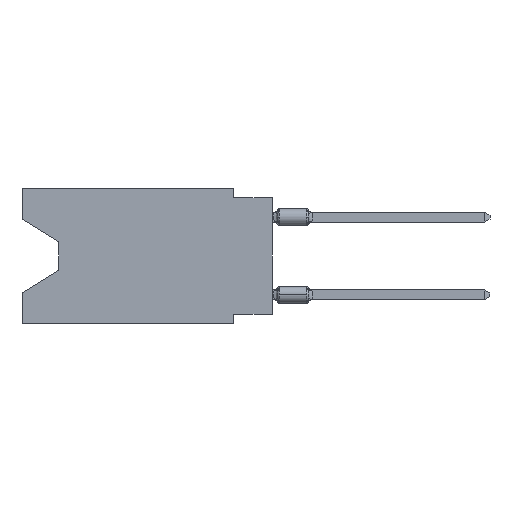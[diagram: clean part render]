
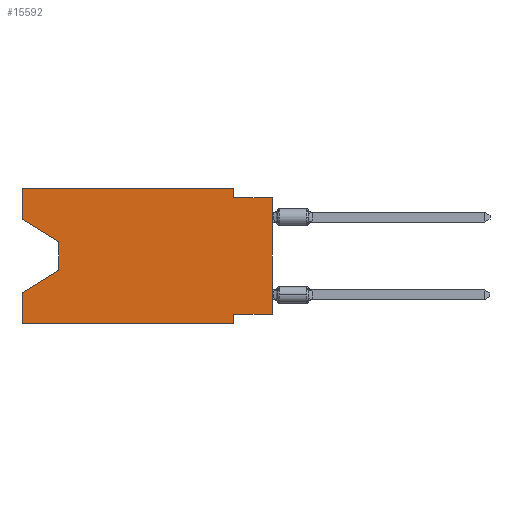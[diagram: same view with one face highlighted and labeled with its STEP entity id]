
A CAD part, left-side view. The second image highlights one B-rep face of the part: STEP entity #15592.
In plain terms, the highlighted planar face has unit normal (-1, 0, 0).
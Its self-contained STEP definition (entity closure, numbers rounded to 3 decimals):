
#167 = VECTOR ( 'NONE', #14594, 1000. ) ;
#469 = LINE ( 'NONE', #5298, #167 ) ;
#749 = CARTESIAN_POINT ( 'NONE',  ( 0., 0., -0.635 ) ) ;
#759 = VERTEX_POINT ( 'NONE', #12636 ) ;
#931 = CARTESIAN_POINT ( 'NONE',  ( 0., 13.97, -5.385 ) ) ;
#1310 = VECTOR ( 'NONE', #17304, 1000. ) ;
#2146 = DIRECTION ( 'NONE',  ( 0., 0.855, -0.519 ) ) ;
#2436 = ORIENTED_EDGE ( 'NONE', *, *, #9040, .F. ) ;
#3117 = CARTESIAN_POINT ( 'NONE',  ( 0., 16.383, 0. ) ) ;
#3445 = LINE ( 'NONE', #17592, #19823 ) ;
#3641 = ORIENTED_EDGE ( 'NONE', *, *, #17355, .F. ) ;
#3659 = VECTOR ( 'NONE', #14726, 1000. ) ;
#3713 = FACE_OUTER_BOUND ( 'NONE', #7505, .T. ) ;
#3949 = ORIENTED_EDGE ( 'NONE', *, *, #13764, .F. ) ;
#4341 = DIRECTION ( 'NONE',  ( 0., 1., 0. ) ) ;
#4489 = ORIENTED_EDGE ( 'NONE', *, *, #13542, .F. ) ;
#4496 = CARTESIAN_POINT ( 'NONE',  ( 0., 2.54, 0. ) ) ;
#4963 = VECTOR ( 'NONE', #6290, 1000. ) ;
#4991 = CARTESIAN_POINT ( 'NONE',  ( 0., 16.383, -2.038 ) ) ;
#5294 = VECTOR ( 'NONE', #7698, 1000. ) ;
#5298 = CARTESIAN_POINT ( 'NONE',  ( 0., 0., -0.635 ) ) ;
#6055 = CARTESIAN_POINT ( 'NONE',  ( 0., 0., -8.255 ) ) ;
#6290 = DIRECTION ( 'NONE',  ( 0., 0., -1. ) ) ;
#6369 = VERTEX_POINT ( 'NONE', #4991 ) ;
#6472 = VECTOR ( 'NONE', #2146, 1000. ) ;
#6800 = ORIENTED_EDGE ( 'NONE', *, *, #13333, .F. ) ;
#6981 = VERTEX_POINT ( 'NONE', #7867 ) ;
#7342 = VECTOR ( 'NONE', #4341, 1000. ) ;
#7441 = CARTESIAN_POINT ( 'NONE',  ( 0., 16.383, -6.852 ) ) ;
#7505 = EDGE_LOOP ( 'NONE', ( #12999, #19137, #13179, #2436, #19481, #6800, #13257, #13892, #3949, #3641, #4489, #15208 ) ) ;
#7665 = VECTOR ( 'NONE', #9278, 1000. ) ;
#7698 = DIRECTION ( 'NONE',  ( 0., 0., -1. ) ) ;
#7867 = CARTESIAN_POINT ( 'NONE',  ( 0., 0., -8.255 ) ) ;
#7872 = CARTESIAN_POINT ( 'NONE',  ( 0., 16.383, -8.89 ) ) ;
#8565 = DIRECTION ( 'NONE',  ( 1., 0., 0. ) ) ;
#8946 = CARTESIAN_POINT ( 'NONE',  ( 0., 16.383, -2.038 ) ) ;
#9040 = EDGE_CURVE ( 'NONE', #12206, #9218, #10771, .T. ) ;
#9218 = VERTEX_POINT ( 'NONE', #7441 ) ;
#9278 = DIRECTION ( 'NONE',  ( 0., 0., 1. ) ) ;
#9312 = LINE ( 'NONE', #15179, #5294 ) ;
#9415 = CARTESIAN_POINT ( 'NONE',  ( 0., 2.54, -8.89 ) ) ;
#9604 = DIRECTION ( 'NONE',  ( 0., -1., 0. ) ) ;
#9686 = PLANE ( 'NONE',  #12420 ) ;
#10248 = LINE ( 'NONE', #8946, #19226 ) ;
#10636 = LINE ( 'NONE', #13659, #4963 ) ;
#10771 = LINE ( 'NONE', #3117, #7665 ) ;
#11118 = LINE ( 'NONE', #12639, #1310 ) ;
#11227 = VECTOR ( 'NONE', #16206, 1000. ) ;
#11413 = LINE ( 'NONE', #931, #6472 ) ;
#11544 = LINE ( 'NONE', #19129, #11227 ) ;
#11802 = VERTEX_POINT ( 'NONE', #17294 ) ;
#12206 = VERTEX_POINT ( 'NONE', #7872 ) ;
#12213 = CARTESIAN_POINT ( 'NONE',  ( 0., 2.54, -0.635 ) ) ;
#12320 = EDGE_CURVE ( 'NONE', #6369, #11802, #15854, .T. ) ;
#12420 = AXIS2_PLACEMENT_3D ( 'NONE', #14531, #8565, #17483 ) ;
#12636 = CARTESIAN_POINT ( 'NONE',  ( 0., 13.97, -5.385 ) ) ;
#12639 = CARTESIAN_POINT ( 'NONE',  ( 0., 0., 0. ) ) ;
#12802 = VERTEX_POINT ( 'NONE', #16220 ) ;
#12965 = EDGE_CURVE ( 'NONE', #17261, #759, #10636, .T. ) ;
#12999 = ORIENTED_EDGE ( 'NONE', *, *, #16183, .T. ) ;
#13179 = ORIENTED_EDGE ( 'NONE', *, *, #19698, .T. ) ;
#13257 = ORIENTED_EDGE ( 'NONE', *, *, #14963, .F. ) ;
#13333 = EDGE_CURVE ( 'NONE', #12802, #16761, #9312, .T. ) ;
#13375 = LINE ( 'NONE', #4496, #17730 ) ;
#13542 = EDGE_CURVE ( 'NONE', #11802, #18433, #3445, .T. ) ;
#13659 = CARTESIAN_POINT ( 'NONE',  ( 0., 13.97, -3.505 ) ) ;
#13764 = EDGE_CURVE ( 'NONE', #18352, #16543, #469, .T. ) ;
#13892 = ORIENTED_EDGE ( 'NONE', *, *, #19581, .T. ) ;
#14531 = CARTESIAN_POINT ( 'NONE',  ( 0., 16.383, 0. ) ) ;
#14594 = DIRECTION ( 'NONE',  ( 0., -1., 0. ) ) ;
#14726 = DIRECTION ( 'NONE',  ( 0., 0., 1. ) ) ;
#14908 = DIRECTION ( 'NONE',  ( 0., -0.855, -0.519 ) ) ;
#14963 = EDGE_CURVE ( 'NONE', #6981, #12802, #18192, .T. ) ;
#15179 = CARTESIAN_POINT ( 'NONE',  ( 0., 2.54, -8.89 ) ) ;
#15208 = ORIENTED_EDGE ( 'NONE', *, *, #12320, .F. ) ;
#15592 = ADVANCED_FACE ( 'NONE', ( #3713 ), #9686, .F. ) ;
#15655 = CARTESIAN_POINT ( 'NONE',  ( 0., 13.97, -3.505 ) ) ;
#15854 = LINE ( 'NONE', #19078, #3659 ) ;
#16183 = EDGE_CURVE ( 'NONE', #6369, #17261, #10248, .T. ) ;
#16206 = DIRECTION ( 'NONE',  ( 0., -1., 0. ) ) ;
#16220 = CARTESIAN_POINT ( 'NONE',  ( 0., 2.54, -8.255 ) ) ;
#16543 = VERTEX_POINT ( 'NONE', #749 ) ;
#16761 = VERTEX_POINT ( 'NONE', #9415 ) ;
#16986 = CARTESIAN_POINT ( 'NONE',  ( 0., 2.54, 0. ) ) ;
#17261 = VERTEX_POINT ( 'NONE', #15655 ) ;
#17294 = CARTESIAN_POINT ( 'NONE',  ( 0., 16.383, 0. ) ) ;
#17304 = DIRECTION ( 'NONE',  ( 0., 0., 1. ) ) ;
#17355 = EDGE_CURVE ( 'NONE', #18433, #18352, #13375, .T. ) ;
#17483 = DIRECTION ( 'NONE',  ( 0., 0., -1. ) ) ;
#17592 = CARTESIAN_POINT ( 'NONE',  ( 0., 16.383, 0. ) ) ;
#17717 = EDGE_CURVE ( 'NONE', #12206, #16761, #11544, .T. ) ;
#17730 = VECTOR ( 'NONE', #19657, 1000. ) ;
#18192 = LINE ( 'NONE', #6055, #7342 ) ;
#18352 = VERTEX_POINT ( 'NONE', #12213 ) ;
#18433 = VERTEX_POINT ( 'NONE', #16986 ) ;
#19078 = CARTESIAN_POINT ( 'NONE',  ( 0., 16.383, 0. ) ) ;
#19129 = CARTESIAN_POINT ( 'NONE',  ( 0., 16.383, -8.89 ) ) ;
#19137 = ORIENTED_EDGE ( 'NONE', *, *, #12965, .T. ) ;
#19226 = VECTOR ( 'NONE', #14908, 1000. ) ;
#19481 = ORIENTED_EDGE ( 'NONE', *, *, #17717, .T. ) ;
#19581 = EDGE_CURVE ( 'NONE', #6981, #16543, #11118, .T. ) ;
#19657 = DIRECTION ( 'NONE',  ( 0., 0., -1. ) ) ;
#19698 = EDGE_CURVE ( 'NONE', #759, #9218, #11413, .T. ) ;
#19823 = VECTOR ( 'NONE', #9604, 1000. ) ;
